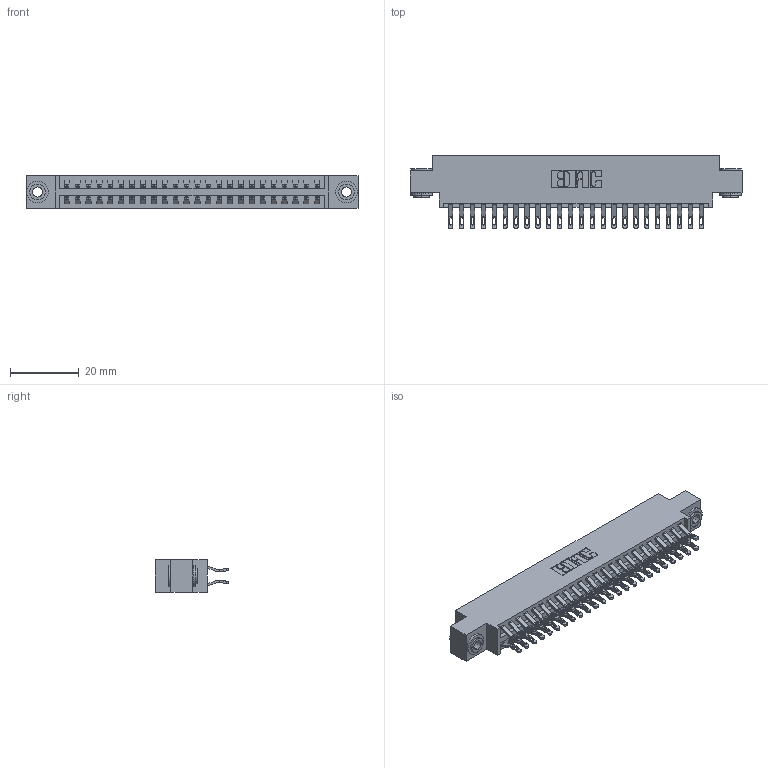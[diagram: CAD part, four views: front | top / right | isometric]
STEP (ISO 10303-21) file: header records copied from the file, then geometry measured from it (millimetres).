
FILE_DESCRIPTION (( 'STEP AP203' ), '1' );
FILE_NAME ('396-048-555-803.STEP', '2019-11-02T07:05:19', ( '' ), ( '' ), 'SwSTEP 2.0', 'SolidWorks 2016', '' );
FILE_SCHEMA (( 'CONFIG_CONTROL_DESIGN' ));
Length unit declared in the file: inch
Products named in the file (4): 345-250-002_345-250-002-102; 396-048-555-803; 346 Part_0.170 Offset - 0.156 Dia-TH; 345-292-001_555 Tail
Assembly tree (51 placements, depth 2):
  396-048-555-803
    346 Part_0.170 Offset - 0.156 Dia-TH
    345-292-001_555 Tail  x48
    345-250-002_345-250-002-102  x2
Bounding box: 96.77 x 21.46 x 9.4 mm (x, y, z)
Volume: 9300.9 mm3; surface area: 13391.9 mm2
Topology: 51 solids, 51 shells, 2948 faces, 9201 edges, 6130 vertices
Faces by surface type: plane 1674, cylinder 1266, cone 8
Entity records: 19194 total; most frequent: CARTESIAN_POINT 3201, ORIENTED_EDGE 3098, DIRECTION 2871, EDGE_CURVE 1549, VECTOR 1277, LINE 1277, VERTEX_POINT 1030, AXIS2_PLACEMENT_3D 797
